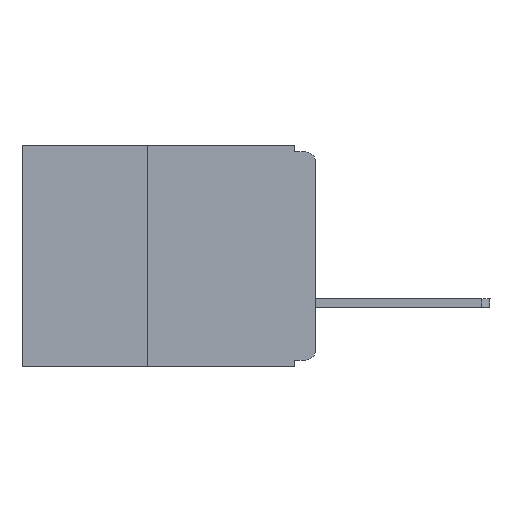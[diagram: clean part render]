
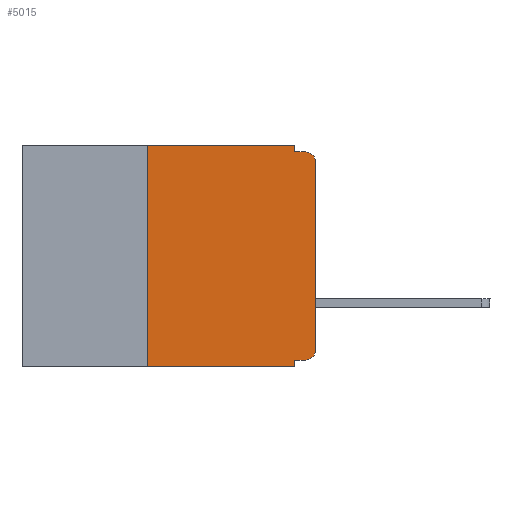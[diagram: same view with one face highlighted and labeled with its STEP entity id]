
A CAD part, left-side view. The second image highlights one B-rep face of the part: STEP entity #5015.
In plain terms, the highlighted planar face has unit normal (-1, 0, 0).
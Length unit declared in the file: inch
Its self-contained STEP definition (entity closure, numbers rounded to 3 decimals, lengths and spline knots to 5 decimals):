
#256 = CARTESIAN_POINT ( 'NONE',  ( 0., 0., -0.305 ) ) ;
#293 = CARTESIAN_POINT ( 'NONE',  ( 0., 0.25, 0. ) ) ;
#362 = VERTEX_POINT ( 'NONE', #7338 ) ;
#553 = VERTEX_POINT ( 'NONE', #6957 ) ;
#613 = CIRCLE ( 'NONE', #4596, 0.015 ) ;
#881 = EDGE_CURVE ( 'NONE', #2028, #5846, #6774, .T. ) ;
#968 = VECTOR ( 'NONE', #3529, 39.37008 ) ;
#998 = CARTESIAN_POINT ( 'NONE',  ( 0., 0.031, -0.33 ) ) ;
#1047 = DIRECTION ( 'NONE',  ( 0., -1., 0. ) ) ;
#1164 = CARTESIAN_POINT ( 'NONE',  ( 0., 0., -0.01 ) ) ;
#1183 = CARTESIAN_POINT ( 'NONE',  ( 0., 0., -0.025 ) ) ;
#1214 = DIRECTION ( 'NONE',  ( 0., 0., -1. ) ) ;
#1295 = DIRECTION ( 'NONE',  ( 0., -1., 0. ) ) ;
#1304 = DIRECTION ( 'NONE',  ( 0., -1., 0. ) ) ;
#1493 = VERTEX_POINT ( 'NONE', #2972 ) ;
#1532 = ORIENTED_EDGE ( 'NONE', *, *, #4640, .F. ) ;
#1535 = ORIENTED_EDGE ( 'NONE', *, *, #881, .T. ) ;
#1631 = VERTEX_POINT ( 'NONE', #9887 ) ;
#1723 = LINE ( 'NONE', #3417, #2249 ) ;
#1910 = CARTESIAN_POINT ( 'NONE',  ( 0., 0.031, 0. ) ) ;
#1978 = ORIENTED_EDGE ( 'NONE', *, *, #9548, .T. ) ;
#2028 = VERTEX_POINT ( 'NONE', #9626 ) ;
#2249 = VECTOR ( 'NONE', #6030, 39.37008 ) ;
#2304 = VECTOR ( 'NONE', #1295, 39.37008 ) ;
#2308 = VECTOR ( 'NONE', #6799, 39.37008 ) ;
#2478 = EDGE_CURVE ( 'NONE', #553, #3648, #4648, .T. ) ;
#2764 = LINE ( 'NONE', #1164, #4737 ) ;
#2870 = ORIENTED_EDGE ( 'NONE', *, *, #8801, .F. ) ;
#2879 = LINE ( 'NONE', #10368, #7470 ) ;
#2972 = CARTESIAN_POINT ( 'NONE',  ( 0., 0.031, 0. ) ) ;
#3417 = CARTESIAN_POINT ( 'NONE',  ( 0., 0., -0.32 ) ) ;
#3529 = DIRECTION ( 'NONE',  ( 0., 0., -1. ) ) ;
#3537 = EDGE_CURVE ( 'NONE', #553, #362, #1723, .T. ) ;
#3648 = VERTEX_POINT ( 'NONE', #256 ) ;
#3754 = LINE ( 'NONE', #6940, #2308 ) ;
#3952 = VECTOR ( 'NONE', #4159, 39.37008 ) ;
#4159 = DIRECTION ( 'NONE',  ( 0., 0., 1. ) ) ;
#4596 = AXIS2_PLACEMENT_3D ( 'NONE', #8777, #5359, #1214 ) ;
#4640 = EDGE_CURVE ( 'NONE', #2028, #8005, #2879, .T. ) ;
#4648 = CIRCLE ( 'NONE', #8653, 0.015 ) ;
#4693 = CARTESIAN_POINT ( 'NONE',  ( 0., 0.437, 0. ) ) ;
#4737 = VECTOR ( 'NONE', #1047, 39.37008 ) ;
#4792 = ORIENTED_EDGE ( 'NONE', *, *, #9802, .F. ) ;
#4905 = ORIENTED_EDGE ( 'NONE', *, *, #6134, .F. ) ;
#5015 = ADVANCED_FACE ( 'NONE', ( #7585 ), #5844, .F. ) ;
#5133 = DIRECTION ( 'NONE',  ( 0., 0., -1. ) ) ;
#5359 = DIRECTION ( 'NONE',  ( -1., 0., 0. ) ) ;
#5365 = DIRECTION ( 'NONE',  ( -1., 0., 0. ) ) ;
#5844 = PLANE ( 'NONE',  #9162 ) ;
#5846 = VERTEX_POINT ( 'NONE', #998 ) ;
#5851 = CARTESIAN_POINT ( 'NONE',  ( 0., 0., 0. ) ) ;
#6030 = DIRECTION ( 'NONE',  ( 0., 1., 0. ) ) ;
#6134 = EDGE_CURVE ( 'NONE', #362, #5846, #3754, .T. ) ;
#6319 = DIRECTION ( 'NONE',  ( 0., 0., -1. ) ) ;
#6455 = LINE ( 'NONE', #5851, #3952 ) ;
#6474 = VERTEX_POINT ( 'NONE', #1183 ) ;
#6477 = EDGE_CURVE ( 'NONE', #6474, #1631, #613, .T. ) ;
#6725 = VECTOR ( 'NONE', #1304, 39.37008 ) ;
#6756 = CARTESIAN_POINT ( 'NONE',  ( 0., 0.437, 0. ) ) ;
#6774 = LINE ( 'NONE', #7896, #2304 ) ;
#6799 = DIRECTION ( 'NONE',  ( 0., 0., -1. ) ) ;
#6939 = ORIENTED_EDGE ( 'NONE', *, *, #6477, .T. ) ;
#6940 = CARTESIAN_POINT ( 'NONE',  ( 0., 0.031, -0.33 ) ) ;
#6957 = CARTESIAN_POINT ( 'NONE',  ( 0., 0.015, -0.32 ) ) ;
#7338 = CARTESIAN_POINT ( 'NONE',  ( 0., 0.031, -0.32 ) ) ;
#7412 = ORIENTED_EDGE ( 'NONE', *, *, #2478, .T. ) ;
#7470 = VECTOR ( 'NONE', #8678, 39.37008 ) ;
#7585 = FACE_OUTER_BOUND ( 'NONE', #9553, .T. ) ;
#7896 = CARTESIAN_POINT ( 'NONE',  ( 0., 0.437, -0.33 ) ) ;
#8005 = VERTEX_POINT ( 'NONE', #293 ) ;
#8101 = VERTEX_POINT ( 'NONE', #10480 ) ;
#8329 = LINE ( 'NONE', #4693, #6725 ) ;
#8559 = EDGE_CURVE ( 'NONE', #1493, #8101, #10385, .T. ) ;
#8563 = ORIENTED_EDGE ( 'NONE', *, *, #8559, .F. ) ;
#8653 = AXIS2_PLACEMENT_3D ( 'NONE', #8855, #5365, #6319 ) ;
#8678 = DIRECTION ( 'NONE',  ( 0., 0., 1. ) ) ;
#8777 = CARTESIAN_POINT ( 'NONE',  ( 0., 0.015, -0.025 ) ) ;
#8801 = EDGE_CURVE ( 'NONE', #8005, #1493, #8329, .T. ) ;
#8855 = CARTESIAN_POINT ( 'NONE',  ( 0., 0.015, -0.305 ) ) ;
#8955 = ORIENTED_EDGE ( 'NONE', *, *, #3537, .F. ) ;
#9162 = AXIS2_PLACEMENT_3D ( 'NONE', #6756, #10138, #5133 ) ;
#9548 = EDGE_CURVE ( 'NONE', #3648, #6474, #6455, .T. ) ;
#9553 = EDGE_LOOP ( 'NONE', ( #1978, #6939, #4792, #8563, #2870, #1532, #1535, #4905, #8955, #7412 ) ) ;
#9626 = CARTESIAN_POINT ( 'NONE',  ( 0., 0.25, -0.33 ) ) ;
#9802 = EDGE_CURVE ( 'NONE', #8101, #1631, #2764, .T. ) ;
#9887 = CARTESIAN_POINT ( 'NONE',  ( 0., 0.015, -0.01 ) ) ;
#10138 = DIRECTION ( 'NONE',  ( 1., 0., 0. ) ) ;
#10368 = CARTESIAN_POINT ( 'NONE',  ( 0., 0.25, -0.33 ) ) ;
#10385 = LINE ( 'NONE', #1910, #968 ) ;
#10480 = CARTESIAN_POINT ( 'NONE',  ( 0., 0.031, -0.01 ) ) ;
